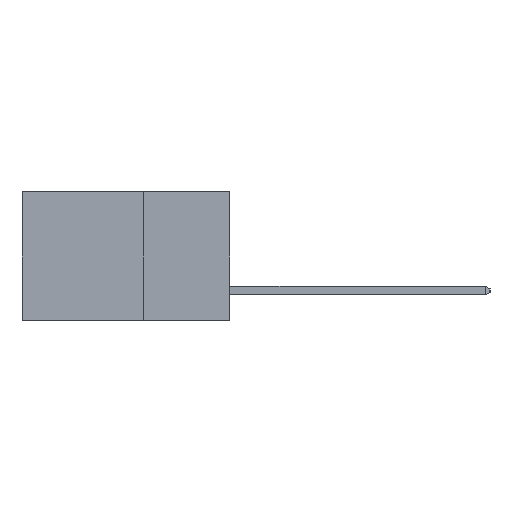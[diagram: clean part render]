
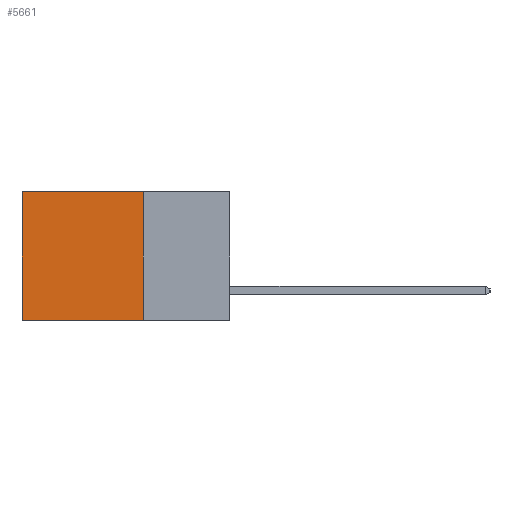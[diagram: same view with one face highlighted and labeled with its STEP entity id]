
A CAD part, left-side view. The second image highlights one B-rep face of the part: STEP entity #5661.
In plain terms, the highlighted planar face has unit normal (-1, 0, 0).
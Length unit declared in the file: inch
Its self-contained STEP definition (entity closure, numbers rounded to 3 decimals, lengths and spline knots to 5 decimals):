
#535 = ORIENTED_EDGE ( 'NONE', *, *, #10368, .F. ) ;
#656 = EDGE_CURVE ( 'NONE', #6199, #6677, #11277, .T. ) ;
#2529 = CARTESIAN_POINT ( 'NONE',  ( 0.2615, 0.6, -0.37 ) ) ;
#2726 = DIRECTION ( 'NONE',  ( 0., 0., -1. ) ) ;
#2753 = DIRECTION ( 'NONE',  ( 1., 0., 0. ) ) ;
#2771 = VECTOR ( 'NONE', #7260, 39.37008 ) ;
#2857 = CARTESIAN_POINT ( 'NONE',  ( 0.2615, 0.6, 0. ) ) ;
#2935 = CARTESIAN_POINT ( 'NONE',  ( 0.2615, 0.25, -0.37 ) ) ;
#2984 = PLANE ( 'NONE',  #4402 ) ;
#3144 = EDGE_LOOP ( 'NONE', ( #8652, #535, #3734, #10446 ) ) ;
#3655 = VERTEX_POINT ( 'NONE', #2857 ) ;
#3734 = ORIENTED_EDGE ( 'NONE', *, *, #656, .F. ) ;
#4402 = AXIS2_PLACEMENT_3D ( 'NONE', #2935, #2753, #2726 ) ;
#4752 = CARTESIAN_POINT ( 'NONE',  ( 0.2615, 0.6, -0.37 ) ) ;
#5158 = DIRECTION ( 'NONE',  ( 0., 1., 0. ) ) ;
#5661 = ADVANCED_FACE ( 'NONE', ( #11519 ), #2984, .F. ) ;
#6199 = VERTEX_POINT ( 'NONE', #10244 ) ;
#6677 = VERTEX_POINT ( 'NONE', #7184 ) ;
#7123 = LINE ( 'NONE', #10754, #9592 ) ;
#7184 = CARTESIAN_POINT ( 'NONE',  ( 0.2615, 0.25, -0.37 ) ) ;
#7240 = VECTOR ( 'NONE', #8187, 39.37008 ) ;
#7260 = DIRECTION ( 'NONE',  ( 0., 1., 0. ) ) ;
#8187 = DIRECTION ( 'NONE',  ( 0., 0., -1. ) ) ;
#8211 = VECTOR ( 'NONE', #8393, 39.37008 ) ;
#8393 = DIRECTION ( 'NONE',  ( 0., 0., -1. ) ) ;
#8582 = EDGE_CURVE ( 'NONE', #3655, #9612, #10005, .T. ) ;
#8652 = ORIENTED_EDGE ( 'NONE', *, *, #8582, .T. ) ;
#8826 = CARTESIAN_POINT ( 'NONE',  ( 0.2615, 0.25, -0.37 ) ) ;
#9076 = CARTESIAN_POINT ( 'NONE',  ( 0.2615, 0.25, 0. ) ) ;
#9592 = VECTOR ( 'NONE', #5158, 39.37008 ) ;
#9612 = VERTEX_POINT ( 'NONE', #4752 ) ;
#10005 = LINE ( 'NONE', #2529, #7240 ) ;
#10244 = CARTESIAN_POINT ( 'NONE',  ( 0.2615, 0.25, 0. ) ) ;
#10276 = LINE ( 'NONE', #9076, #2771 ) ;
#10368 = EDGE_CURVE ( 'NONE', #6677, #9612, #7123, .T. ) ;
#10446 = ORIENTED_EDGE ( 'NONE', *, *, #12201, .T. ) ;
#10754 = CARTESIAN_POINT ( 'NONE',  ( 0.2615, 0.25, -0.37 ) ) ;
#11277 = LINE ( 'NONE', #8826, #8211 ) ;
#11519 = FACE_OUTER_BOUND ( 'NONE', #3144, .T. ) ;
#12201 = EDGE_CURVE ( 'NONE', #6199, #3655, #10276, .T. ) ;
